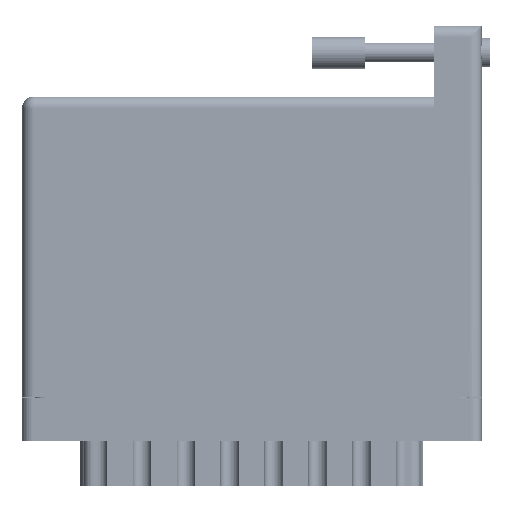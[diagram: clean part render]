
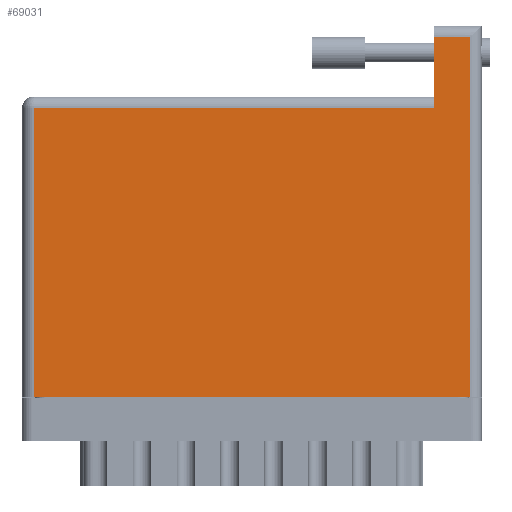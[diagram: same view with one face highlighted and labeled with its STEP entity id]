
A CAD part, front view. The second image highlights one B-rep face of the part: STEP entity #69031.
In plain terms, the highlighted face is planar.
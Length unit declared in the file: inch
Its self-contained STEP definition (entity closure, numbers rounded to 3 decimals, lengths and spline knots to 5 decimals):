
#1728 = VERTEX_POINT ( 'NONE', #8932 ) ;
#4704 = LINE ( 'NONE', #9879, #48466 ) ;
#7620 = LINE ( 'NONE', #30107, #55982 ) ;
#8368 = DIRECTION ( 'NONE',  ( 0., -1., 0. ) ) ;
#8932 = CARTESIAN_POINT ( 'NONE',  ( 2.438, 2.125, 0. ) ) ;
#9879 = CARTESIAN_POINT ( 'NONE',  ( 0., 1.705, 0. ) ) ;
#10977 = CARTESIAN_POINT ( 'NONE',  ( 0.07, 1.705, 0. ) ) ;
#11966 = VERTEX_POINT ( 'NONE', #47455 ) ;
#12348 = VECTOR ( 'NONE', #34071, 39.37008 ) ;
#12561 = PLANE ( 'NONE',  #62454 ) ;
#13073 = ORIENTED_EDGE ( 'NONE', *, *, #66231, .T. ) ;
#13980 = VECTOR ( 'NONE', #36546, 39.37008 ) ;
#18817 = DIRECTION ( 'NONE',  ( 0., -1., 0. ) ) ;
#19167 = ORIENTED_EDGE ( 'NONE', *, *, #56954, .T. ) ;
#21396 = EDGE_LOOP ( 'NONE', ( #70980, #19167, #30904, #46757, #72409, #13073 ) ) ;
#23261 = DIRECTION ( 'NONE',  ( -1., 0., 0. ) ) ;
#24838 = EDGE_CURVE ( 'NONE', #11966, #1728, #37280, .T. ) ;
#25255 = VECTOR ( 'NONE', #8368, 39.37008 ) ;
#28898 = CARTESIAN_POINT ( 'NONE',  ( 0., 0., 0. ) ) ;
#30107 = CARTESIAN_POINT ( 'NONE',  ( 2.648, 2.195, 0. ) ) ;
#30904 = ORIENTED_EDGE ( 'NONE', *, *, #34379, .T. ) ;
#31274 = VERTEX_POINT ( 'NONE', #69672 ) ;
#34071 = DIRECTION ( 'NONE',  ( 1., 0., 0. ) ) ;
#34379 = EDGE_CURVE ( 'NONE', #62307, #56198, #40701, .T. ) ;
#35406 = FACE_OUTER_BOUND ( 'NONE', #21396, .T. ) ;
#36546 = DIRECTION ( 'NONE',  ( -1., 0., 0. ) ) ;
#37280 = LINE ( 'NONE', #64139, #13980 ) ;
#38971 = CARTESIAN_POINT ( 'NONE',  ( 0.07, 0., 0. ) ) ;
#40605 = LINE ( 'NONE', #46845, #43369 ) ;
#40701 = LINE ( 'NONE', #28898, #12348 ) ;
#40823 = DIRECTION ( 'NONE',  ( 0., 1., 0. ) ) ;
#43369 = VECTOR ( 'NONE', #18817, 39.37008 ) ;
#44204 = VERTEX_POINT ( 'NONE', #10977 ) ;
#46666 = EDGE_CURVE ( 'NONE', #56198, #11966, #7620, .T. ) ;
#46757 = ORIENTED_EDGE ( 'NONE', *, *, #46666, .T. ) ;
#46845 = CARTESIAN_POINT ( 'NONE',  ( 2.438, 2.195, 0. ) ) ;
#47455 = CARTESIAN_POINT ( 'NONE',  ( 2.648, 2.125, 0. ) ) ;
#48466 = VECTOR ( 'NONE', #54837, 39.37008 ) ;
#48565 = CARTESIAN_POINT ( 'NONE',  ( 0.07, 0., 0. ) ) ;
#48812 = CARTESIAN_POINT ( 'NONE',  ( 2.648, 0., 0. ) ) ;
#51266 = DIRECTION ( 'NONE',  ( 0., 0., -1. ) ) ;
#54109 = EDGE_CURVE ( 'NONE', #31274, #44204, #4704, .T. ) ;
#54837 = DIRECTION ( 'NONE',  ( -1., 0., 0. ) ) ;
#55982 = VECTOR ( 'NONE', #40823, 39.37008 ) ;
#56198 = VERTEX_POINT ( 'NONE', #48812 ) ;
#56954 = EDGE_CURVE ( 'NONE', #44204, #62307, #58852, .T. ) ;
#57854 = CARTESIAN_POINT ( 'NONE',  ( 0., 1.775, 0. ) ) ;
#58852 = LINE ( 'NONE', #48565, #25255 ) ;
#62307 = VERTEX_POINT ( 'NONE', #38971 ) ;
#62454 = AXIS2_PLACEMENT_3D ( 'NONE', #57854, #51266, #23261 ) ;
#64139 = CARTESIAN_POINT ( 'NONE',  ( 0., 2.125, 0. ) ) ;
#66231 = EDGE_CURVE ( 'NONE', #1728, #31274, #40605, .T. ) ;
#69031 = ADVANCED_FACE ( 'NONE', ( #35406 ), #12561, .F. ) ;
#69672 = CARTESIAN_POINT ( 'NONE',  ( 2.438, 1.705, 0. ) ) ;
#70980 = ORIENTED_EDGE ( 'NONE', *, *, #54109, .T. ) ;
#72409 = ORIENTED_EDGE ( 'NONE', *, *, #24838, .T. ) ;
